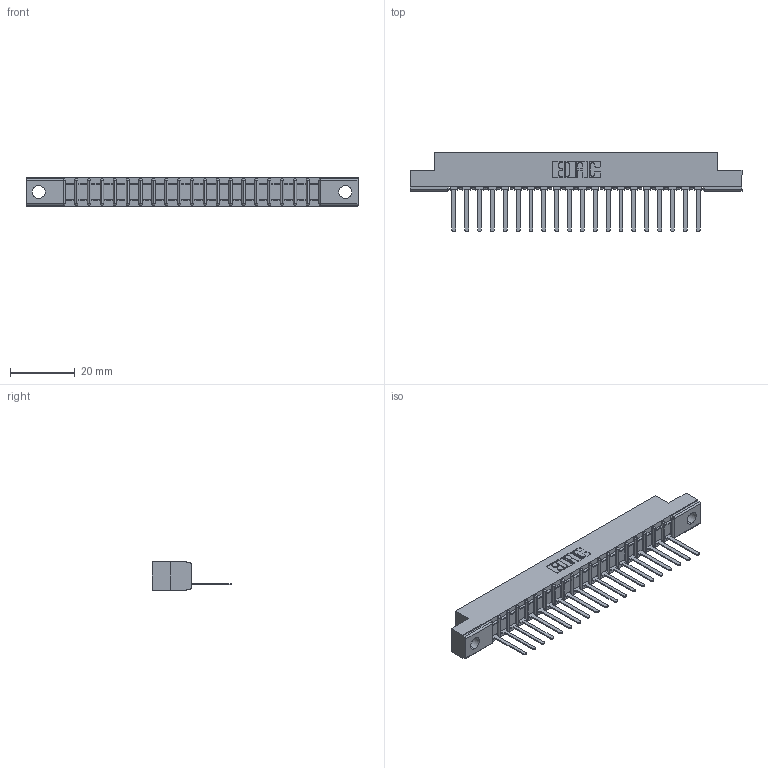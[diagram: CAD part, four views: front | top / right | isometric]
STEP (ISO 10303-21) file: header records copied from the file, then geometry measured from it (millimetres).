
FILE_DESCRIPTION (( 'STEP AP203' ), '1' );
FILE_NAME ('307-020-441-102.STEP', '2020-09-27T02:47:19', ( '' ), ( '' ), 'SwSTEP 2.0', 'SolidWorks 2020', '' );
FILE_SCHEMA (( 'CONFIG_CONTROL_DESIGN' ));
Length unit declared in the file: inch
Products named in the file (3): 307-020-441-102; 307-290-002_541; 307 Part_.128 Dia Mounting Holes
Assembly tree (21 placements, depth 2):
  307-020-441-102
    307 Part_.128 Dia Mounting Holes
    307-290-002_541  x20
Bounding box: 102.26 x 24.59 x 8.71 mm (x, y, z)
Volume: 6718.6 mm3; surface area: 12297.8 mm2
Topology: 21 solids, 21 shells, 1619 faces, 4963 edges, 3250 vertices
Faces by surface type: plane 970, cylinder 607, sphere 42
Entity records: 20578 total; most frequent: CARTESIAN_POINT 3468, ORIENTED_EDGE 3458, DIRECTION 3379, EDGE_CURVE 1729, LINE 1313, VECTOR 1313, VERTEX_POINT 1122, AXIS2_PLACEMENT_3D 1033
